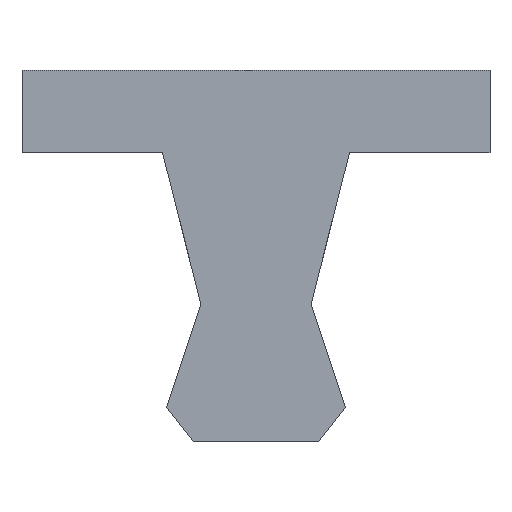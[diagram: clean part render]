
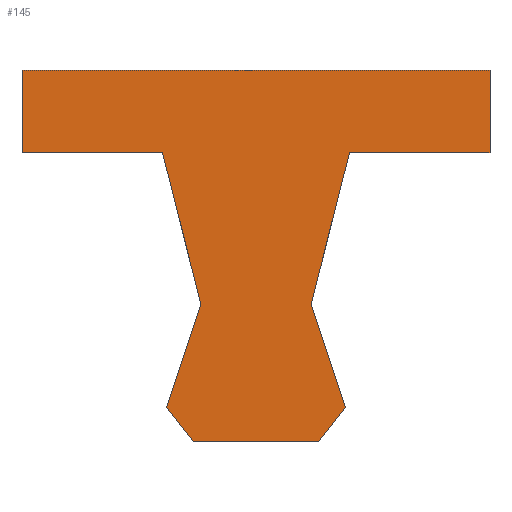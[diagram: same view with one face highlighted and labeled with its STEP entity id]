
A CAD part, top view. The second image highlights one B-rep face of the part: STEP entity #145.
In plain terms, the highlighted planar face has unit normal (0, 0, 1).
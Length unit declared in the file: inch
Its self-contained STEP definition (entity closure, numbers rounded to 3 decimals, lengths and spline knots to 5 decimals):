
#3 = VERTEX_POINT ( 'NONE', #390 ) ;
#5 = EDGE_CURVE ( 'NONE', #148, #154, #241, .T. ) ;
#9 = CARTESIAN_POINT ( 'NONE',  ( 0.065, -0.245, 0.024 ) ) ;
#12 = LINE ( 'NONE', #324, #216 ) ;
#13 = EDGE_CURVE ( 'NONE', #32, #3, #384, .T. ) ;
#19 = CARTESIAN_POINT ( 'NONE',  ( 0., 0., 0.024 ) ) ;
#25 = EDGE_CURVE ( 'NONE', #3, #442, #355, .T. ) ;
#32 = VERTEX_POINT ( 'NONE', #200 ) ;
#33 = EDGE_CURVE ( 'NONE', #442, #300, #322, .T. ) ;
#39 = ORIENTED_EDGE ( 'NONE', *, *, #13, .T. ) ;
#41 = ORIENTED_EDGE ( 'NONE', *, *, #339, .T. ) ;
#43 = VECTOR ( 'NONE', #427, 39.37008 ) ;
#45 = EDGE_LOOP ( 'NONE', ( #39, #410, #349, #230, #408, #224, #82, #41, #374, #352, #439, #407 ) ) ;
#47 = VERTEX_POINT ( 'NONE', #453 ) ;
#51 = CARTESIAN_POINT ( 'NONE',  ( -0.0455, -0.27, 0.024 ) ) ;
#52 = CARTESIAN_POINT ( 'NONE',  ( -0.17, -0.06, 0.024 ) ) ;
#53 = EDGE_CURVE ( 'NONE', #269, #32, #173, .T. ) ;
#54 = LINE ( 'NONE', #132, #470 ) ;
#55 = DIRECTION ( 'NONE',  ( 1., 0., 0. ) ) ;
#57 = LINE ( 'NONE', #205, #231 ) ;
#69 = CARTESIAN_POINT ( 'NONE',  ( -0.068, -0.06, 0.024 ) ) ;
#71 = EDGE_CURVE ( 'NONE', #77, #314, #257, .T. ) ;
#77 = VERTEX_POINT ( 'NONE', #283 ) ;
#82 = ORIENTED_EDGE ( 'NONE', *, *, #194, .T. ) ;
#95 = DIRECTION ( 'NONE',  ( 0.247, -0.969, 0. ) ) ;
#100 = DIRECTION ( 'NONE',  ( 0., 1., 0. ) ) ;
#102 = CARTESIAN_POINT ( 'NONE',  ( -0.17, 0., 0.024 ) ) ;
#112 = VECTOR ( 'NONE', #95, 39.37008 ) ;
#118 = EDGE_CURVE ( 'NONE', #300, #47, #57, .T. ) ;
#132 = CARTESIAN_POINT ( 'NONE',  ( 0.17, -0.06, 0.024 ) ) ;
#133 = DIRECTION ( 'NONE',  ( 0.247, 0.969, 0. ) ) ;
#145 = ADVANCED_FACE ( 'NONE', ( #357 ), #265, .T. ) ;
#148 = VERTEX_POINT ( 'NONE', #51 ) ;
#154 = VERTEX_POINT ( 'NONE', #454 ) ;
#169 = DIRECTION ( 'NONE',  ( 0., -1., 0. ) ) ;
#173 = LINE ( 'NONE', #102, #181 ) ;
#181 = VECTOR ( 'NONE', #325, 39.37008 ) ;
#194 = EDGE_CURVE ( 'NONE', #154, #366, #383, .T. ) ;
#197 = EDGE_CURVE ( 'NONE', #47, #148, #240, .T. ) ;
#198 = CARTESIAN_POINT ( 'NONE',  ( 0.17, 0., 0.024 ) ) ;
#200 = CARTESIAN_POINT ( 'NONE',  ( -0.17, 0., 0.024 ) ) ;
#205 = CARTESIAN_POINT ( 'NONE',  ( -0.04, -0.17, 0.024 ) ) ;
#208 = VERTEX_POINT ( 'NONE', #248 ) ;
#216 = VECTOR ( 'NONE', #450, 39.37008 ) ;
#220 = CARTESIAN_POINT ( 'NONE',  ( -0.065, -0.245, 0.024 ) ) ;
#224 = ORIENTED_EDGE ( 'NONE', *, *, #5, .T. ) ;
#230 = ORIENTED_EDGE ( 'NONE', *, *, #118, .T. ) ;
#231 = VECTOR ( 'NONE', #351, 39.37008 ) ;
#240 = LINE ( 'NONE', #220, #473 ) ;
#241 = LINE ( 'NONE', #387, #413 ) ;
#245 = CARTESIAN_POINT ( 'NONE',  ( -0.04, -0.17, 0.024 ) ) ;
#247 = VECTOR ( 'NONE', #100, 39.37008 ) ;
#248 = CARTESIAN_POINT ( 'NONE',  ( 0.17, -0.06, 0.024 ) ) ;
#249 = CARTESIAN_POINT ( 'NONE',  ( 0.068, -0.06, 0.024 ) ) ;
#257 = LINE ( 'NONE', #360, #409 ) ;
#264 = EDGE_CURVE ( 'NONE', #208, #269, #394, .T. ) ;
#265 = PLANE ( 'NONE',  #469 ) ;
#269 = VERTEX_POINT ( 'NONE', #198 ) ;
#280 = DIRECTION ( 'NONE',  ( 0., 0., 1. ) ) ;
#281 = CARTESIAN_POINT ( 'NONE',  ( -0.068, -0.06, 0.024 ) ) ;
#283 = CARTESIAN_POINT ( 'NONE',  ( 0.04, -0.17, 0.024 ) ) ;
#292 = CARTESIAN_POINT ( 'NONE',  ( 0.17, 0., 0.024 ) ) ;
#300 = VERTEX_POINT ( 'NONE', #245 ) ;
#313 = CARTESIAN_POINT ( 'NONE',  ( 0.065, -0.245, 0.024 ) ) ;
#314 = VERTEX_POINT ( 'NONE', #249 ) ;
#322 = LINE ( 'NONE', #281, #112 ) ;
#324 = CARTESIAN_POINT ( 'NONE',  ( 0.04, -0.17, 0.024 ) ) ;
#325 = DIRECTION ( 'NONE',  ( -1., 0., 0. ) ) ;
#328 = DIRECTION ( 'NONE',  ( 0.615, -0.789, 0. ) ) ;
#339 = EDGE_CURVE ( 'NONE', #366, #77, #12, .T. ) ;
#349 = ORIENTED_EDGE ( 'NONE', *, *, #33, .T. ) ;
#351 = DIRECTION ( 'NONE',  ( -0.316, -0.949, 0. ) ) ;
#352 = ORIENTED_EDGE ( 'NONE', *, *, #364, .T. ) ;
#353 = DIRECTION ( 'NONE',  ( 1., 0., 0. ) ) ;
#355 = LINE ( 'NONE', #52, #431 ) ;
#357 = FACE_OUTER_BOUND ( 'NONE', #45, .T. ) ;
#358 = CARTESIAN_POINT ( 'NONE',  ( -0.17, 0., 0.024 ) ) ;
#360 = CARTESIAN_POINT ( 'NONE',  ( 0.068, -0.06, 0.024 ) ) ;
#364 = EDGE_CURVE ( 'NONE', #314, #208, #54, .T. ) ;
#366 = VERTEX_POINT ( 'NONE', #9 ) ;
#374 = ORIENTED_EDGE ( 'NONE', *, *, #71, .T. ) ;
#379 = VECTOR ( 'NONE', #169, 39.37008 ) ;
#383 = LINE ( 'NONE', #313, #43 ) ;
#384 = LINE ( 'NONE', #358, #379 ) ;
#386 = DIRECTION ( 'NONE',  ( 1., 0., 0. ) ) ;
#387 = CARTESIAN_POINT ( 'NONE',  ( -0.0455, -0.27, 0.024 ) ) ;
#390 = CARTESIAN_POINT ( 'NONE',  ( -0.17, -0.06, 0.024 ) ) ;
#394 = LINE ( 'NONE', #292, #247 ) ;
#407 = ORIENTED_EDGE ( 'NONE', *, *, #53, .T. ) ;
#408 = ORIENTED_EDGE ( 'NONE', *, *, #197, .T. ) ;
#409 = VECTOR ( 'NONE', #133, 39.37008 ) ;
#410 = ORIENTED_EDGE ( 'NONE', *, *, #25, .T. ) ;
#413 = VECTOR ( 'NONE', #55, 39.37008 ) ;
#427 = DIRECTION ( 'NONE',  ( 0.615, 0.789, 0. ) ) ;
#431 = VECTOR ( 'NONE', #456, 39.37008 ) ;
#439 = ORIENTED_EDGE ( 'NONE', *, *, #264, .T. ) ;
#442 = VERTEX_POINT ( 'NONE', #69 ) ;
#450 = DIRECTION ( 'NONE',  ( -0.316, 0.949, 0. ) ) ;
#453 = CARTESIAN_POINT ( 'NONE',  ( -0.065, -0.245, 0.024 ) ) ;
#454 = CARTESIAN_POINT ( 'NONE',  ( 0.0455, -0.27, 0.024 ) ) ;
#456 = DIRECTION ( 'NONE',  ( 1., 0., 0. ) ) ;
#469 = AXIS2_PLACEMENT_3D ( 'NONE', #19, #280, #386 ) ;
#470 = VECTOR ( 'NONE', #353, 39.37008 ) ;
#473 = VECTOR ( 'NONE', #328, 39.37008 ) ;
